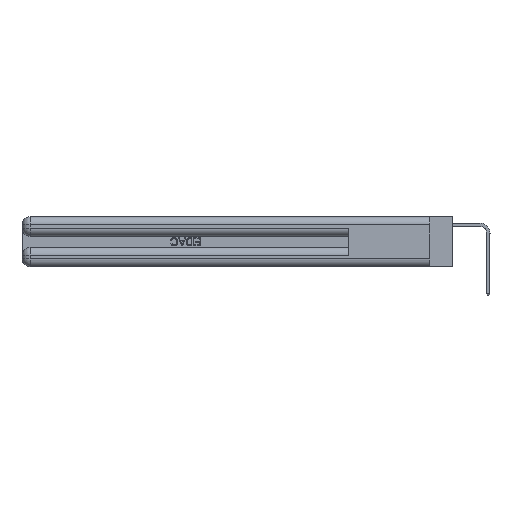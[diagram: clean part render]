
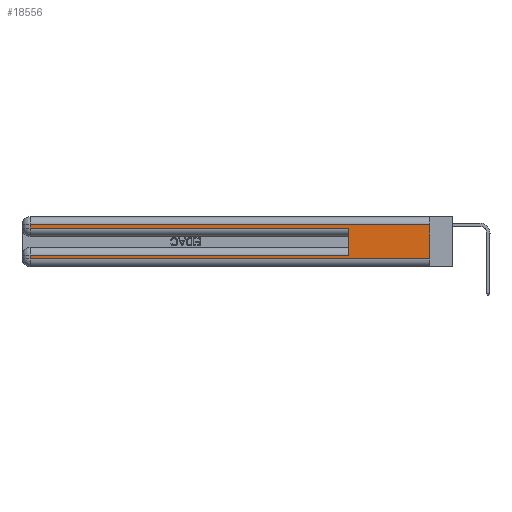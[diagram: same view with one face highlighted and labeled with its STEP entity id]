
A CAD part, left-side view. The second image highlights one B-rep face of the part: STEP entity #18556.
In plain terms, the highlighted planar face has unit normal (-1, 0, 0).
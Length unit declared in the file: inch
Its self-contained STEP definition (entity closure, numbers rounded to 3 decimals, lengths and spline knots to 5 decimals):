
#966 = CARTESIAN_POINT ( 'NONE',  ( 0., 0., 0.06 ) ) ;
#1283 = LINE ( 'NONE', #18760, #25612 ) ;
#1752 = DIRECTION ( 'NONE',  ( 0., 0., -1. ) ) ;
#1891 = EDGE_CURVE ( 'NONE', #25745, #16958, #1283, .T. ) ;
#1995 = VECTOR ( 'NONE', #27450, 39.37008 ) ;
#3064 = VERTEX_POINT ( 'NONE', #11259 ) ;
#3402 = DIRECTION ( 'NONE',  ( 0., -1., 0. ) ) ;
#3508 = EDGE_CURVE ( 'NONE', #25745, #14463, #7664, .T. ) ;
#4039 = LINE ( 'NONE', #6671, #12031 ) ;
#4633 = CARTESIAN_POINT ( 'NONE',  ( 0., 0., 0.285 ) ) ;
#6671 = CARTESIAN_POINT ( 'NONE',  ( 0., 2.94, 0.37 ) ) ;
#7052 = VERTEX_POINT ( 'NONE', #14731 ) ;
#7481 = AXIS2_PLACEMENT_3D ( 'NONE', #21105, #31044, #16518 ) ;
#7664 = LINE ( 'NONE', #20157, #1995 ) ;
#10036 = EDGE_CURVE ( 'NONE', #14463, #7052, #4039, .T. ) ;
#10469 = ORIENTED_EDGE ( 'NONE', *, *, #3508, .T. ) ;
#11259 = CARTESIAN_POINT ( 'NONE',  ( 0., 2.94, 0.06 ) ) ;
#11414 = CARTESIAN_POINT ( 'NONE',  ( 0., 0.6, 0.145 ) ) ;
#11572 = LINE ( 'NONE', #11414, #23737 ) ;
#11666 = EDGE_CURVE ( 'NONE', #7052, #21981, #13136, .T. ) ;
#11908 = DIRECTION ( 'NONE',  ( 0., 1., 0. ) ) ;
#12031 = VECTOR ( 'NONE', #23702, 39.37008 ) ;
#12043 = LINE ( 'NONE', #966, #17736 ) ;
#12394 = VECTOR ( 'NONE', #24082, 39.37008 ) ;
#12577 = VERTEX_POINT ( 'NONE', #30058 ) ;
#12704 = CARTESIAN_POINT ( 'NONE',  ( 0., 2.94, 0.085 ) ) ;
#13136 = LINE ( 'NONE', #4633, #12394 ) ;
#13291 = EDGE_CURVE ( 'NONE', #12577, #21981, #11572, .T. ) ;
#13294 = ORIENTED_EDGE ( 'NONE', *, *, #19813, .T. ) ;
#13941 = DIRECTION ( 'NONE',  ( 0., 0., 1. ) ) ;
#14075 = PLANE ( 'NONE',  #7481 ) ;
#14463 = VERTEX_POINT ( 'NONE', #26412 ) ;
#14731 = CARTESIAN_POINT ( 'NONE',  ( 0., 2.94, 0.285 ) ) ;
#15506 = ORIENTED_EDGE ( 'NONE', *, *, #13291, .F. ) ;
#16518 = DIRECTION ( 'NONE',  ( 0., 0., -1. ) ) ;
#16709 = ORIENTED_EDGE ( 'NONE', *, *, #10036, .T. ) ;
#16958 = VERTEX_POINT ( 'NONE', #18108 ) ;
#17736 = VECTOR ( 'NONE', #3402, 39.37008 ) ;
#18108 = CARTESIAN_POINT ( 'NONE',  ( 0., 0., 0.06 ) ) ;
#18556 = ADVANCED_FACE ( 'NONE', ( #30011 ), #14075, .F. ) ;
#18738 = ORIENTED_EDGE ( 'NONE', *, *, #1891, .F. ) ;
#18760 = CARTESIAN_POINT ( 'NONE',  ( 0., 0., 0.37 ) ) ;
#19813 = EDGE_CURVE ( 'NONE', #12577, #27920, #21268, .T. ) ;
#20157 = CARTESIAN_POINT ( 'NONE',  ( 0., 0., 0.31 ) ) ;
#20301 = LINE ( 'NONE', #27322, #30909 ) ;
#21105 = CARTESIAN_POINT ( 'NONE',  ( 0., 0., 0.37 ) ) ;
#21268 = LINE ( 'NONE', #24129, #28482 ) ;
#21436 = EDGE_CURVE ( 'NONE', #3064, #16958, #12043, .T. ) ;
#21981 = VERTEX_POINT ( 'NONE', #30127 ) ;
#22972 = ORIENTED_EDGE ( 'NONE', *, *, #23060, .T. ) ;
#23060 = EDGE_CURVE ( 'NONE', #27920, #3064, #20301, .T. ) ;
#23702 = DIRECTION ( 'NONE',  ( 0., 0., -1. ) ) ;
#23737 = VECTOR ( 'NONE', #13941, 39.37008 ) ;
#24082 = DIRECTION ( 'NONE',  ( 0., -1., 0. ) ) ;
#24129 = CARTESIAN_POINT ( 'NONE',  ( 0., 0., 0.085 ) ) ;
#24963 = ORIENTED_EDGE ( 'NONE', *, *, #11666, .T. ) ;
#25249 = CARTESIAN_POINT ( 'NONE',  ( 0., 0., 0.31 ) ) ;
#25612 = VECTOR ( 'NONE', #1752, 39.37008 ) ;
#25745 = VERTEX_POINT ( 'NONE', #25249 ) ;
#26412 = CARTESIAN_POINT ( 'NONE',  ( 0., 2.94, 0.31 ) ) ;
#27322 = CARTESIAN_POINT ( 'NONE',  ( 0., 2.94, 0.37 ) ) ;
#27450 = DIRECTION ( 'NONE',  ( 0., 1., 0. ) ) ;
#27920 = VERTEX_POINT ( 'NONE', #12704 ) ;
#28482 = VECTOR ( 'NONE', #11908, 39.37008 ) ;
#29760 = DIRECTION ( 'NONE',  ( 0., 0., -1. ) ) ;
#29839 = ORIENTED_EDGE ( 'NONE', *, *, #21436, .T. ) ;
#30011 = FACE_OUTER_BOUND ( 'NONE', #30406, .T. ) ;
#30058 = CARTESIAN_POINT ( 'NONE',  ( 0., 0.6, 0.085 ) ) ;
#30127 = CARTESIAN_POINT ( 'NONE',  ( 0., 0.6, 0.285 ) ) ;
#30406 = EDGE_LOOP ( 'NONE', ( #18738, #10469, #16709, #24963, #15506, #13294, #22972, #29839 ) ) ;
#30909 = VECTOR ( 'NONE', #29760, 39.37008 ) ;
#31044 = DIRECTION ( 'NONE',  ( 1., 0., 0. ) ) ;
